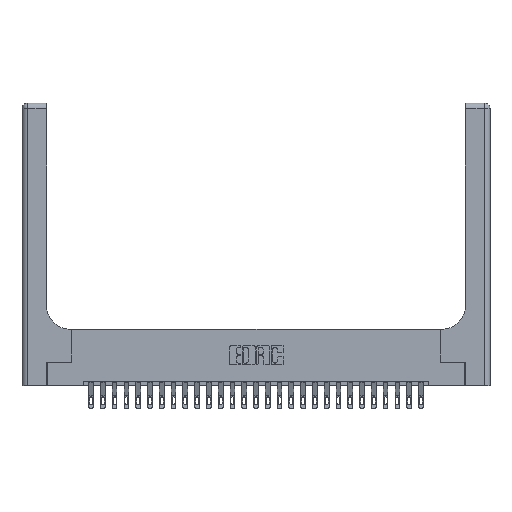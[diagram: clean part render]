
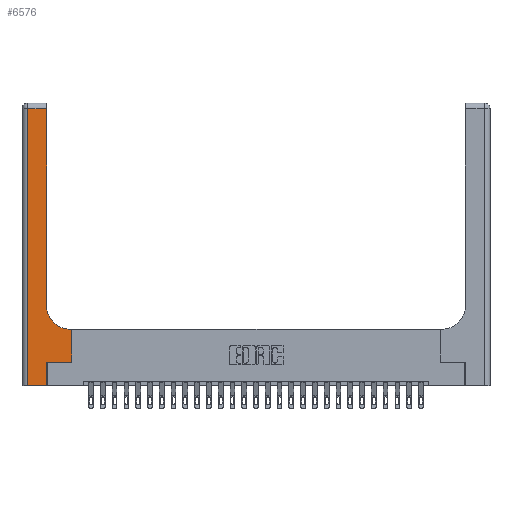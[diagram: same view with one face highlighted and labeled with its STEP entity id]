
A CAD part, top view. The second image highlights one B-rep face of the part: STEP entity #6576.
In plain terms, the highlighted planar face has unit normal (0, 0, 1).
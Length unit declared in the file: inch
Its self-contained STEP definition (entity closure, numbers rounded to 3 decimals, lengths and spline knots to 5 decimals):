
#156 = ORIENTED_EDGE ( 'NONE', *, *, #21386, .T. ) ;
#183 = ORIENTED_EDGE ( 'NONE', *, *, #17935, .T. ) ;
#2371 = CARTESIAN_POINT ( 'NONE',  ( 0.528, 0.6, 0.37 ) ) ;
#3098 = EDGE_CURVE ( 'NONE', #23854, #16102, #22110, .T. ) ;
#3537 = CARTESIAN_POINT ( 'NONE',  ( 0.26, 3., 0.37 ) ) ;
#4194 = CARTESIAN_POINT ( 'NONE',  ( 0.265, 0., 0.37 ) ) ;
#4732 = AXIS2_PLACEMENT_3D ( 'NONE', #6252, #9894, #10162 ) ;
#5185 = ORIENTED_EDGE ( 'NONE', *, *, #22584, .T. ) ;
#5425 = CARTESIAN_POINT ( 'NONE',  ( 0.265, 0.25, 0.37 ) ) ;
#5813 = VERTEX_POINT ( 'NONE', #8576 ) ;
#5839 = CARTESIAN_POINT ( 'NONE',  ( 0.26, 0.6, 0.37 ) ) ;
#5879 = ORIENTED_EDGE ( 'NONE', *, *, #21754, .T. ) ;
#5948 = VECTOR ( 'NONE', #18968, 39.37008 ) ;
#6252 = CARTESIAN_POINT ( 'NONE',  ( 0.51, 0.85, 0.37 ) ) ;
#6576 = ADVANCED_FACE ( 'NONE', ( #18809 ), #12590, .F. ) ;
#6638 = VECTOR ( 'NONE', #20139, 39.37008 ) ;
#7656 = CARTESIAN_POINT ( 'NONE',  ( 0., 2.94, 0.37 ) ) ;
#7880 = LINE ( 'NONE', #24038, #6638 ) ;
#8014 = DIRECTION ( 'NONE',  ( -1., 0., 0. ) ) ;
#8414 = DIRECTION ( 'NONE',  ( 0., 0., -1. ) ) ;
#8576 = CARTESIAN_POINT ( 'NONE',  ( 0.26, 0.85, 0.37 ) ) ;
#8853 = VERTEX_POINT ( 'NONE', #13306 ) ;
#9478 = AXIS2_PLACEMENT_3D ( 'NONE', #24573, #8414, #16637 ) ;
#9894 = DIRECTION ( 'NONE',  ( 0., 0., -1. ) ) ;
#9914 = CARTESIAN_POINT ( 'NONE',  ( 0.265, 0.25, 0.37 ) ) ;
#9971 = VECTOR ( 'NONE', #10135, 39.37008 ) ;
#10135 = DIRECTION ( 'NONE',  ( 0., 1., 0. ) ) ;
#10158 = CARTESIAN_POINT ( 'NONE',  ( 0.51, 0.6, 0.37 ) ) ;
#10162 = DIRECTION ( 'NONE',  ( 1., 0., 0. ) ) ;
#11213 = CIRCLE ( 'NONE', #4732, 0.25 ) ;
#11903 = LINE ( 'NONE', #3537, #12841 ) ;
#12077 = CARTESIAN_POINT ( 'NONE',  ( 0.06, 2.94, 0.37 ) ) ;
#12546 = VECTOR ( 'NONE', #8014, 39.37008 ) ;
#12590 = PLANE ( 'NONE',  #9478 ) ;
#12841 = VECTOR ( 'NONE', #26056, 39.37008 ) ;
#13179 = VERTEX_POINT ( 'NONE', #15956 ) ;
#13306 = CARTESIAN_POINT ( 'NONE',  ( 0.265, 0., 0.37 ) ) ;
#13309 = VERTEX_POINT ( 'NONE', #10158 ) ;
#13395 = VERTEX_POINT ( 'NONE', #21578 ) ;
#13667 = DIRECTION ( 'NONE',  ( 1., 0., 0. ) ) ;
#15020 = EDGE_CURVE ( 'NONE', #13179, #23862, #21788, .T. ) ;
#15102 = LINE ( 'NONE', #23171, #25567 ) ;
#15788 = EDGE_CURVE ( 'NONE', #5813, #13179, #11903, .T. ) ;
#15956 = CARTESIAN_POINT ( 'NONE',  ( 0.26, 2.94, 0.37 ) ) ;
#16102 = VERTEX_POINT ( 'NONE', #23684 ) ;
#16637 = DIRECTION ( 'NONE',  ( -1., 0., 0. ) ) ;
#17254 = VECTOR ( 'NONE', #13667, 39.37008 ) ;
#17295 = EDGE_LOOP ( 'NONE', ( #19543, #18374, #183, #20197, #5879, #19384, #5185, #156, #25458 ) ) ;
#17935 = EDGE_CURVE ( 'NONE', #23862, #13395, #19084, .T. ) ;
#17984 = VERTEX_POINT ( 'NONE', #2371 ) ;
#18374 = ORIENTED_EDGE ( 'NONE', *, *, #15020, .T. ) ;
#18809 = FACE_OUTER_BOUND ( 'NONE', #17295, .T. ) ;
#18968 = DIRECTION ( 'NONE',  ( 0., -1., 0. ) ) ;
#19084 = LINE ( 'NONE', #21078, #5948 ) ;
#19384 = ORIENTED_EDGE ( 'NONE', *, *, #3098, .T. ) ;
#19543 = ORIENTED_EDGE ( 'NONE', *, *, #15788, .T. ) ;
#20098 = EDGE_CURVE ( 'NONE', #13309, #5813, #11213, .T. ) ;
#20139 = DIRECTION ( 'NONE',  ( 0., 1., 0. ) ) ;
#20197 = ORIENTED_EDGE ( 'NONE', *, *, #24476, .T. ) ;
#21078 = CARTESIAN_POINT ( 'NONE',  ( 0.06, 3., 0.37 ) ) ;
#21386 = EDGE_CURVE ( 'NONE', #17984, #13309, #26474, .T. ) ;
#21578 = CARTESIAN_POINT ( 'NONE',  ( 0.06, 0., 0.37 ) ) ;
#21754 = EDGE_CURVE ( 'NONE', #8853, #23854, #22516, .T. ) ;
#21788 = LINE ( 'NONE', #7656, #21800 ) ;
#21800 = VECTOR ( 'NONE', #21922, 39.37008 ) ;
#21922 = DIRECTION ( 'NONE',  ( -1., 0., 0. ) ) ;
#22110 = LINE ( 'NONE', #5425, #17254 ) ;
#22516 = LINE ( 'NONE', #4194, #9971 ) ;
#22584 = EDGE_CURVE ( 'NONE', #16102, #17984, #7880, .T. ) ;
#23171 = CARTESIAN_POINT ( 'NONE',  ( 0., 0., 0.37 ) ) ;
#23300 = DIRECTION ( 'NONE',  ( 1., 0., 0. ) ) ;
#23684 = CARTESIAN_POINT ( 'NONE',  ( 0.528, 0.25, 0.37 ) ) ;
#23854 = VERTEX_POINT ( 'NONE', #9914 ) ;
#23862 = VERTEX_POINT ( 'NONE', #12077 ) ;
#24038 = CARTESIAN_POINT ( 'NONE',  ( 0.528, 0.25, 0.37 ) ) ;
#24476 = EDGE_CURVE ( 'NONE', #13395, #8853, #15102, .T. ) ;
#24573 = CARTESIAN_POINT ( 'NONE',  ( 0., 3., 0.37 ) ) ;
#25458 = ORIENTED_EDGE ( 'NONE', *, *, #20098, .T. ) ;
#25567 = VECTOR ( 'NONE', #23300, 39.37008 ) ;
#26056 = DIRECTION ( 'NONE',  ( 0., 1., 0. ) ) ;
#26474 = LINE ( 'NONE', #5839, #12546 ) ;
